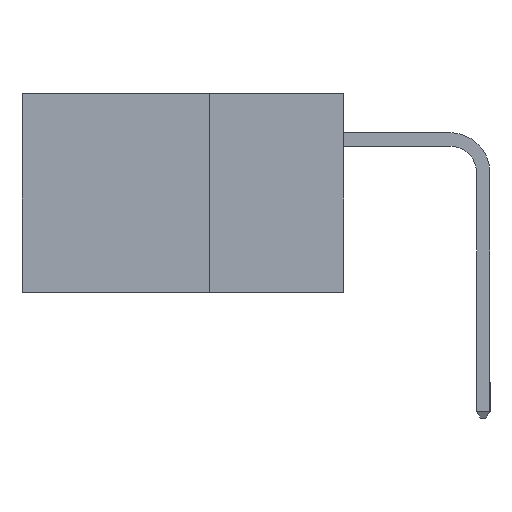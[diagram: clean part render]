
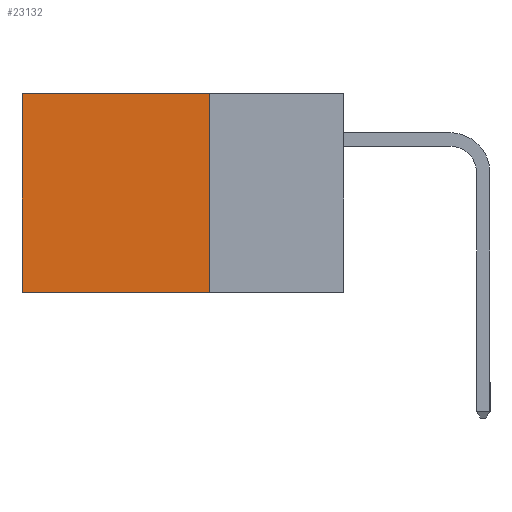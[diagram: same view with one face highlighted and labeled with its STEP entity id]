
A CAD part, left-side view. The second image highlights one B-rep face of the part: STEP entity #23132.
In plain terms, the highlighted planar face has unit normal (-1, 0, 0).
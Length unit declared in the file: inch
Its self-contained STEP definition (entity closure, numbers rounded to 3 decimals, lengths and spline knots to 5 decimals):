
#166 = CARTESIAN_POINT ( 'NONE',  ( 0.298, 0.25, 0. ) ) ;
#267 = CARTESIAN_POINT ( 'NONE',  ( 0.298, 0.25, -0.37 ) ) ;
#1971 = ORIENTED_EDGE ( 'NONE', *, *, #26224, .F. ) ;
#2411 = EDGE_CURVE ( 'NONE', #17392, #17030, #16285, .T. ) ;
#2556 = DIRECTION ( 'NONE',  ( 0., 0., -1. ) ) ;
#3537 = CARTESIAN_POINT ( 'NONE',  ( 0.298, 0.6, -0.37 ) ) ;
#4776 = VECTOR ( 'NONE', #26207, 39.37008 ) ;
#5318 = VECTOR ( 'NONE', #15222, 39.37008 ) ;
#5512 = ORIENTED_EDGE ( 'NONE', *, *, #24179, .T. ) ;
#6018 = CARTESIAN_POINT ( 'NONE',  ( 0.298, 0.25, -0.37 ) ) ;
#6726 = CARTESIAN_POINT ( 'NONE',  ( 0.298, 0.25, 0. ) ) ;
#6884 = LINE ( 'NONE', #6018, #4776 ) ;
#9261 = PLANE ( 'NONE',  #9946 ) ;
#9946 = AXIS2_PLACEMENT_3D ( 'NONE', #166, #15793, #2556 ) ;
#10101 = CARTESIAN_POINT ( 'NONE',  ( 0.298, 0.25, 0. ) ) ;
#11855 = DIRECTION ( 'NONE',  ( 0., 0., -1. ) ) ;
#12562 = FACE_OUTER_BOUND ( 'NONE', #22331, .T. ) ;
#13545 = ORIENTED_EDGE ( 'NONE', *, *, #13815, .T. ) ;
#13805 = VECTOR ( 'NONE', #11855, 39.37008 ) ;
#13815 = EDGE_CURVE ( 'NONE', #19905, #20097, #19554, .T. ) ;
#14934 = CARTESIAN_POINT ( 'NONE',  ( 0.298, 0.25, 0. ) ) ;
#15222 = DIRECTION ( 'NONE',  ( 0., 0., -1. ) ) ;
#15793 = DIRECTION ( 'NONE',  ( 1., 0., 0. ) ) ;
#16285 = LINE ( 'NONE', #6726, #5318 ) ;
#17030 = VERTEX_POINT ( 'NONE', #267 ) ;
#17392 = VERTEX_POINT ( 'NONE', #14934 ) ;
#17946 = VECTOR ( 'NONE', #25047, 39.37008 ) ;
#19554 = LINE ( 'NONE', #22540, #13805 ) ;
#19905 = VERTEX_POINT ( 'NONE', #26211 ) ;
#20097 = VERTEX_POINT ( 'NONE', #3537 ) ;
#22331 = EDGE_LOOP ( 'NONE', ( #13545, #1971, #23615, #5512 ) ) ;
#22540 = CARTESIAN_POINT ( 'NONE',  ( 0.298, 0.6, 0. ) ) ;
#23132 = ADVANCED_FACE ( 'NONE', ( #12562 ), #9261, .F. ) ;
#23548 = LINE ( 'NONE', #10101, #17946 ) ;
#23615 = ORIENTED_EDGE ( 'NONE', *, *, #2411, .F. ) ;
#24179 = EDGE_CURVE ( 'NONE', #17392, #19905, #23548, .T. ) ;
#25047 = DIRECTION ( 'NONE',  ( 0., 1., 0. ) ) ;
#26207 = DIRECTION ( 'NONE',  ( 0., 1., 0. ) ) ;
#26211 = CARTESIAN_POINT ( 'NONE',  ( 0.298, 0.6, 0. ) ) ;
#26224 = EDGE_CURVE ( 'NONE', #17030, #20097, #6884, .T. ) ;
